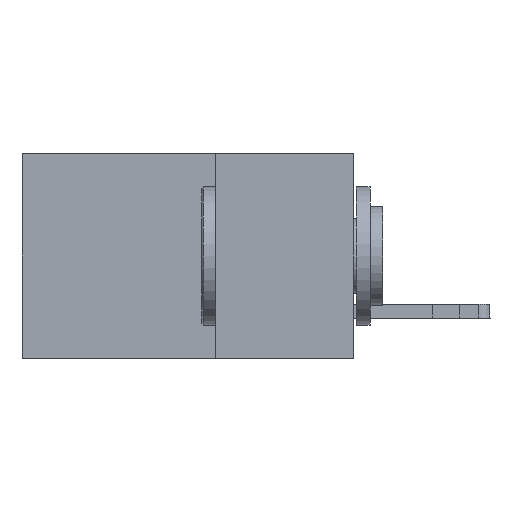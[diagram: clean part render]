
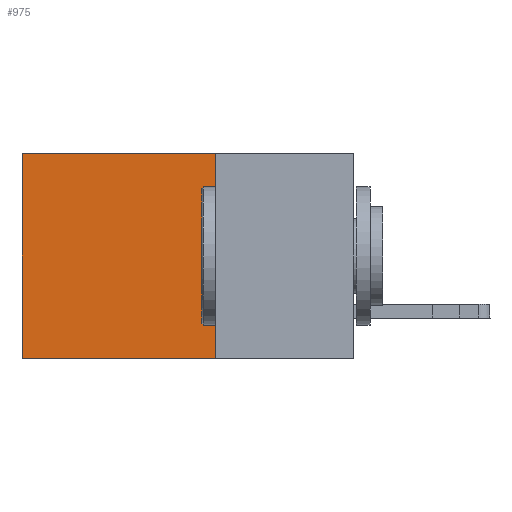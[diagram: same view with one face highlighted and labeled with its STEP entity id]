
A CAD part, left-side view. The second image highlights one B-rep face of the part: STEP entity #975.
In plain terms, the highlighted planar face has unit normal (-1, 0, 0).
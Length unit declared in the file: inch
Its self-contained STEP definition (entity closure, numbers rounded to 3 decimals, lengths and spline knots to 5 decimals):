
#92 = VECTOR ( 'NONE', #10108, 39.37008 ) ;
#161 = ORIENTED_EDGE ( 'NONE', *, *, #1268, .T. ) ;
#535 = CARTESIAN_POINT ( 'NONE',  ( 0.2875, 0.25, -0.37 ) ) ;
#897 = ORIENTED_EDGE ( 'NONE', *, *, #5918, .F. ) ;
#975 = ADVANCED_FACE ( 'NONE', ( #18549 ), #8682, .F. ) ;
#1268 = EDGE_CURVE ( 'NONE', #9817, #6610, #6089, .T. ) ;
#1797 = LINE ( 'NONE', #14642, #5308 ) ;
#2416 = CARTESIAN_POINT ( 'NONE',  ( 0.2875, 0.25, 0. ) ) ;
#2887 = LINE ( 'NONE', #15408, #18179 ) ;
#3348 = EDGE_CURVE ( 'NONE', #4163, #9817, #16026, .T. ) ;
#4163 = VERTEX_POINT ( 'NONE', #2416 ) ;
#4362 = VERTEX_POINT ( 'NONE', #535 ) ;
#5308 = VECTOR ( 'NONE', #5652, 39.37008 ) ;
#5652 = DIRECTION ( 'NONE',  ( 0., 1., 0. ) ) ;
#5758 = CARTESIAN_POINT ( 'NONE',  ( 0.2875, 0.6, -0.37 ) ) ;
#5918 = EDGE_CURVE ( 'NONE', #4163, #4362, #2887, .T. ) ;
#6089 = LINE ( 'NONE', #8634, #17454 ) ;
#6610 = VERTEX_POINT ( 'NONE', #5758 ) ;
#7097 = ORIENTED_EDGE ( 'NONE', *, *, #3348, .T. ) ;
#8542 = DIRECTION ( 'NONE',  ( 0., 0., -1. ) ) ;
#8567 = DIRECTION ( 'NONE',  ( 1., 0., 0. ) ) ;
#8571 = CARTESIAN_POINT ( 'NONE',  ( 0.2875, 0.25, 0. ) ) ;
#8634 = CARTESIAN_POINT ( 'NONE',  ( 0.2875, 0.6, 0. ) ) ;
#8682 = PLANE ( 'NONE',  #12449 ) ;
#9817 = VERTEX_POINT ( 'NONE', #14083 ) ;
#10108 = DIRECTION ( 'NONE',  ( 0., 1., 0. ) ) ;
#10127 = CARTESIAN_POINT ( 'NONE',  ( 0.2875, 0.25, 0. ) ) ;
#10574 = ORIENTED_EDGE ( 'NONE', *, *, #16817, .F. ) ;
#12269 = EDGE_LOOP ( 'NONE', ( #161, #10574, #897, #7097 ) ) ;
#12449 = AXIS2_PLACEMENT_3D ( 'NONE', #8571, #8567, #8542 ) ;
#12768 = DIRECTION ( 'NONE',  ( 0., 0., -1. ) ) ;
#14083 = CARTESIAN_POINT ( 'NONE',  ( 0.2875, 0.6, 0. ) ) ;
#14642 = CARTESIAN_POINT ( 'NONE',  ( 0.2875, 0.25, -0.37 ) ) ;
#15408 = CARTESIAN_POINT ( 'NONE',  ( 0.2875, 0.25, 0. ) ) ;
#15572 = DIRECTION ( 'NONE',  ( 0., 0., -1. ) ) ;
#16026 = LINE ( 'NONE', #10127, #92 ) ;
#16817 = EDGE_CURVE ( 'NONE', #4362, #6610, #1797, .T. ) ;
#17454 = VECTOR ( 'NONE', #12768, 39.37008 ) ;
#18179 = VECTOR ( 'NONE', #15572, 39.37008 ) ;
#18549 = FACE_OUTER_BOUND ( 'NONE', #12269, .T. ) ;
